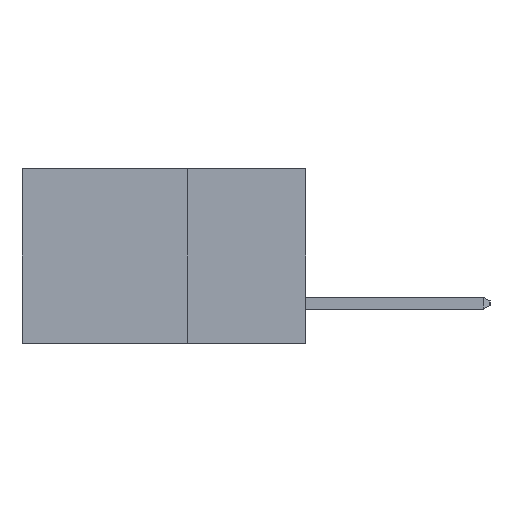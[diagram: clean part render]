
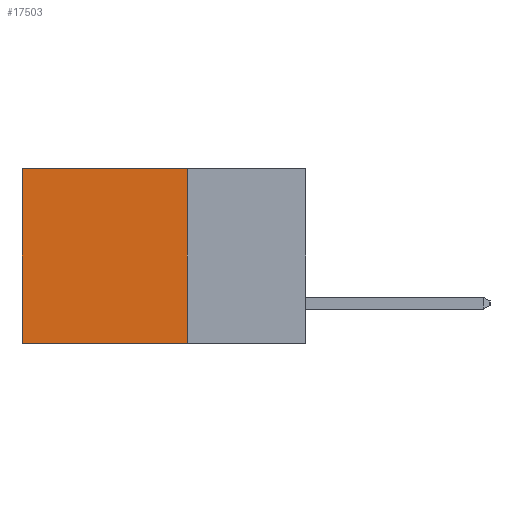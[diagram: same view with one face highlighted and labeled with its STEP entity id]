
A CAD part, left-side view. The second image highlights one B-rep face of the part: STEP entity #17503.
In plain terms, the highlighted planar face has unit normal (-1, 0, 0).
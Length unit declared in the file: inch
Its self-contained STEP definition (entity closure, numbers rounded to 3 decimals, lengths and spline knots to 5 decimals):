
#2440 = LINE ( 'NONE', #10302, #7640 ) ;
#3751 = LINE ( 'NONE', #5588, #20822 ) ;
#5240 = CARTESIAN_POINT ( 'NONE',  ( 0.298, 0.25, -0.37 ) ) ;
#5588 = CARTESIAN_POINT ( 'NONE',  ( 0.298, 0.25, 0. ) ) ;
#6434 = EDGE_CURVE ( 'NONE', #8316, #19856, #2440, .T. ) ;
#7305 = PLANE ( 'NONE',  #28039 ) ;
#7640 = VECTOR ( 'NONE', #16991, 39.37008 ) ;
#7788 = DIRECTION ( 'NONE',  ( 0., 0., -1. ) ) ;
#7988 = VECTOR ( 'NONE', #10580, 39.37008 ) ;
#8316 = VERTEX_POINT ( 'NONE', #19840 ) ;
#9533 = DIRECTION ( 'NONE',  ( 1., 0., 0. ) ) ;
#10302 = CARTESIAN_POINT ( 'NONE',  ( 0.298, 0.6, 0. ) ) ;
#10580 = DIRECTION ( 'NONE',  ( 0., 1., 0. ) ) ;
#10788 = VERTEX_POINT ( 'NONE', #15286 ) ;
#11691 = EDGE_LOOP ( 'NONE', ( #26749, #23619, #27253, #26242 ) ) ;
#12800 = EDGE_CURVE ( 'NONE', #10788, #16756, #3751, .T. ) ;
#14174 = EDGE_CURVE ( 'NONE', #10788, #8316, #17811, .T. ) ;
#15286 = CARTESIAN_POINT ( 'NONE',  ( 0.298, 0.25, 0. ) ) ;
#16004 = CARTESIAN_POINT ( 'NONE',  ( 0.298, 0.25, 0. ) ) ;
#16756 = VERTEX_POINT ( 'NONE', #5240 ) ;
#16991 = DIRECTION ( 'NONE',  ( 0., 0., -1. ) ) ;
#17182 = CARTESIAN_POINT ( 'NONE',  ( 0.298, 0.25, -0.37 ) ) ;
#17503 = ADVANCED_FACE ( 'NONE', ( #27998 ), #7305, .F. ) ;
#17681 = CARTESIAN_POINT ( 'NONE',  ( 0.298, 0.6, -0.37 ) ) ;
#17811 = LINE ( 'NONE', #16004, #24440 ) ;
#19840 = CARTESIAN_POINT ( 'NONE',  ( 0.298, 0.6, 0. ) ) ;
#19856 = VERTEX_POINT ( 'NONE', #17681 ) ;
#20822 = VECTOR ( 'NONE', #7788, 39.37008 ) ;
#23435 = EDGE_CURVE ( 'NONE', #16756, #19856, #26427, .T. ) ;
#23619 = ORIENTED_EDGE ( 'NONE', *, *, #23435, .F. ) ;
#24440 = VECTOR ( 'NONE', #24888, 39.37008 ) ;
#24888 = DIRECTION ( 'NONE',  ( 0., 1., 0. ) ) ;
#25110 = DIRECTION ( 'NONE',  ( 0., 0., -1. ) ) ;
#26242 = ORIENTED_EDGE ( 'NONE', *, *, #14174, .T. ) ;
#26427 = LINE ( 'NONE', #17182, #7988 ) ;
#26749 = ORIENTED_EDGE ( 'NONE', *, *, #6434, .T. ) ;
#27227 = CARTESIAN_POINT ( 'NONE',  ( 0.298, 0.25, 0. ) ) ;
#27253 = ORIENTED_EDGE ( 'NONE', *, *, #12800, .F. ) ;
#27998 = FACE_OUTER_BOUND ( 'NONE', #11691, .T. ) ;
#28039 = AXIS2_PLACEMENT_3D ( 'NONE', #27227, #9533, #25110 ) ;
